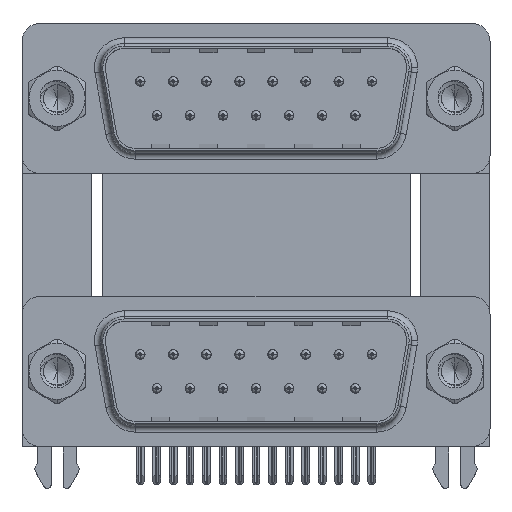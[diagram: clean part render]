
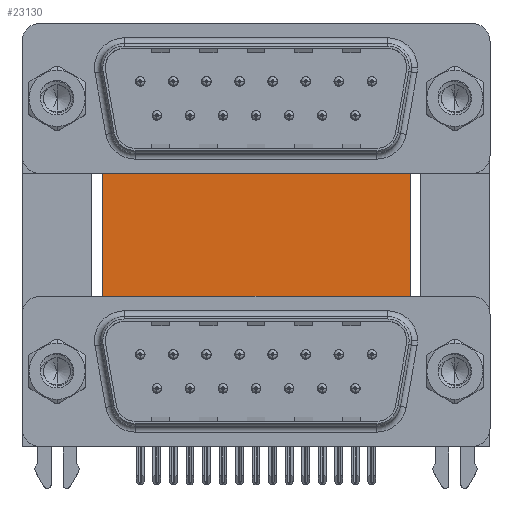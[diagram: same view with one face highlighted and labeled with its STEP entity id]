
A CAD part, top view. The second image highlights one B-rep face of the part: STEP entity #23130.
In plain terms, the highlighted planar face has unit normal (0, 0, 1).
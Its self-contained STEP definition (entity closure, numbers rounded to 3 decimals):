
#679 = VECTOR ( 'NONE', #9049, 1000. ) ;
#1072 = ORIENTED_EDGE ( 'NONE', *, *, #16639, .F. ) ;
#1410 = AXIS2_PLACEMENT_3D ( 'NONE', #5636, #32171, #35499 ) ;
#3139 = LINE ( 'NONE', #35951, #679 ) ;
#3163 = ORIENTED_EDGE ( 'NONE', *, *, #15402, .T. ) ;
#4961 = CARTESIAN_POINT ( 'NONE',  ( 3.79, -3.735, -12. ) ) ;
#5244 = FACE_OUTER_BOUND ( 'NONE', #27793, .T. ) ;
#5636 = CARTESIAN_POINT ( 'NONE',  ( 3.79, 16.585, -12. ) ) ;
#9049 = DIRECTION ( 'NONE',  ( 1., 0., 0. ) ) ;
#9343 = CARTESIAN_POINT ( 'NONE',  ( 29.58, -3.735, -12. ) ) ;
#9735 = DIRECTION ( 'NONE',  ( 1., 0., 0. ) ) ;
#11141 = VERTEX_POINT ( 'NONE', #17654 ) ;
#11158 = VERTEX_POINT ( 'NONE', #11183 ) ;
#11183 = CARTESIAN_POINT ( 'NONE',  ( 3.79, 16.585, -12. ) ) ;
#15402 = EDGE_CURVE ( 'NONE', #11158, #20856, #32997, .T. ) ;
#16639 = EDGE_CURVE ( 'NONE', #11158, #11141, #3139, .T. ) ;
#17442 = CARTESIAN_POINT ( 'NONE',  ( 29.58, 16.585, -12. ) ) ;
#17654 = CARTESIAN_POINT ( 'NONE',  ( 29.58, 16.585, -12. ) ) ;
#17820 = PLANE ( 'NONE',  #1410 ) ;
#18807 = VECTOR ( 'NONE', #32804, 1000. ) ;
#19247 = EDGE_CURVE ( 'NONE', #20856, #27740, #36644, .T. ) ;
#20856 = VERTEX_POINT ( 'NONE', #4961 ) ;
#21497 = VECTOR ( 'NONE', #9735, 1000. ) ;
#22945 = LINE ( 'NONE', #17442, #28594 ) ;
#23130 = ADVANCED_FACE ( 'NONE', ( #5244 ), #17820, .F. ) ;
#24146 = CARTESIAN_POINT ( 'NONE',  ( 3.79, 16.585, -12. ) ) ;
#27740 = VERTEX_POINT ( 'NONE', #9343 ) ;
#27793 = EDGE_LOOP ( 'NONE', ( #36616, #37746, #1072, #3163 ) ) ;
#27984 = CARTESIAN_POINT ( 'NONE',  ( 3.79, -3.735, -12. ) ) ;
#28594 = VECTOR ( 'NONE', #29422, 1000. ) ;
#29422 = DIRECTION ( 'NONE',  ( 0., -1., 0. ) ) ;
#32171 = DIRECTION ( 'NONE',  ( 0., 0., -1. ) ) ;
#32804 = DIRECTION ( 'NONE',  ( 0., -1., 0. ) ) ;
#32997 = LINE ( 'NONE', #24146, #18807 ) ;
#35499 = DIRECTION ( 'NONE',  ( -1., 0., 0. ) ) ;
#35951 = CARTESIAN_POINT ( 'NONE',  ( 3.79, 16.585, -12. ) ) ;
#36616 = ORIENTED_EDGE ( 'NONE', *, *, #19247, .T. ) ;
#36644 = LINE ( 'NONE', #27984, #21497 ) ;
#37052 = EDGE_CURVE ( 'NONE', #11141, #27740, #22945, .T. ) ;
#37746 = ORIENTED_EDGE ( 'NONE', *, *, #37052, .F. ) ;
